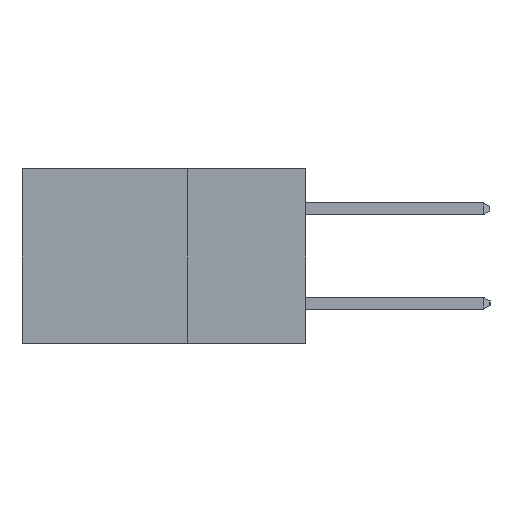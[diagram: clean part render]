
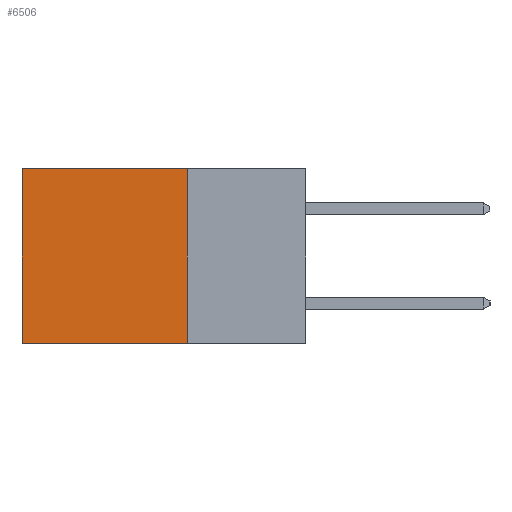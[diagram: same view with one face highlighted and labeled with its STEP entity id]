
A CAD part, left-side view. The second image highlights one B-rep face of the part: STEP entity #6506.
In plain terms, the highlighted planar face has unit normal (-1, 0, 0).
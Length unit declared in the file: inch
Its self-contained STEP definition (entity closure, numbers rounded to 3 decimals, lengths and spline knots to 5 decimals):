
#39 = DIRECTION ( 'NONE',  ( 0., 0., -1. ) ) ;
#42 = DIRECTION ( 'NONE',  ( 1., 0., 0. ) ) ;
#62 = CARTESIAN_POINT ( 'NONE',  ( 0.2615, 0.25, -0.37 ) ) ;
#207 = EDGE_CURVE ( 'NONE', #13698, #6234, #17456, .T. ) ;
#946 = PLANE ( 'NONE',  #16491 ) ;
#1183 = ORIENTED_EDGE ( 'NONE', *, *, #8918, .T. ) ;
#2437 = ORIENTED_EDGE ( 'NONE', *, *, #6171, .F. ) ;
#2566 = VECTOR ( 'NONE', #5710, 39.37008 ) ;
#5608 = VERTEX_POINT ( 'NONE', #10241 ) ;
#5648 = VERTEX_POINT ( 'NONE', #7475 ) ;
#5710 = DIRECTION ( 'NONE',  ( 0., 1., 0. ) ) ;
#5778 = CARTESIAN_POINT ( 'NONE',  ( 0.2615, 0.25, 0. ) ) ;
#5779 = EDGE_LOOP ( 'NONE', ( #14745, #8595, #2437, #1183 ) ) ;
#5853 = DIRECTION ( 'NONE',  ( 0., 1., 0. ) ) ;
#6171 = EDGE_CURVE ( 'NONE', #5608, #13698, #16757, .T. ) ;
#6234 = VERTEX_POINT ( 'NONE', #7602 ) ;
#6506 = ADVANCED_FACE ( 'NONE', ( #19159 ), #946, .F. ) ;
#6719 = CARTESIAN_POINT ( 'NONE',  ( 0.2615, 0.25, -0.37 ) ) ;
#7045 = DIRECTION ( 'NONE',  ( 0., 0., -1. ) ) ;
#7064 = LINE ( 'NONE', #13382, #14995 ) ;
#7316 = LINE ( 'NONE', #5778, #2566 ) ;
#7475 = CARTESIAN_POINT ( 'NONE',  ( 0.2615, 0.6, 0. ) ) ;
#7602 = CARTESIAN_POINT ( 'NONE',  ( 0.2615, 0.6, -0.37 ) ) ;
#8312 = CARTESIAN_POINT ( 'NONE',  ( 0.2615, 0.25, -0.37 ) ) ;
#8361 = VECTOR ( 'NONE', #8879, 39.37008 ) ;
#8595 = ORIENTED_EDGE ( 'NONE', *, *, #207, .F. ) ;
#8879 = DIRECTION ( 'NONE',  ( 0., 0., -1. ) ) ;
#8918 = EDGE_CURVE ( 'NONE', #5608, #5648, #7316, .T. ) ;
#9066 = VECTOR ( 'NONE', #5853, 39.37008 ) ;
#10241 = CARTESIAN_POINT ( 'NONE',  ( 0.2615, 0.25, 0. ) ) ;
#11060 = CARTESIAN_POINT ( 'NONE',  ( 0.2615, 0.25, -0.37 ) ) ;
#13382 = CARTESIAN_POINT ( 'NONE',  ( 0.2615, 0.6, -0.37 ) ) ;
#13698 = VERTEX_POINT ( 'NONE', #6719 ) ;
#14585 = EDGE_CURVE ( 'NONE', #5648, #6234, #7064, .T. ) ;
#14745 = ORIENTED_EDGE ( 'NONE', *, *, #14585, .T. ) ;
#14995 = VECTOR ( 'NONE', #7045, 39.37008 ) ;
#16491 = AXIS2_PLACEMENT_3D ( 'NONE', #62, #42, #39 ) ;
#16757 = LINE ( 'NONE', #8312, #8361 ) ;
#17456 = LINE ( 'NONE', #11060, #9066 ) ;
#19159 = FACE_OUTER_BOUND ( 'NONE', #5779, .T. ) ;
